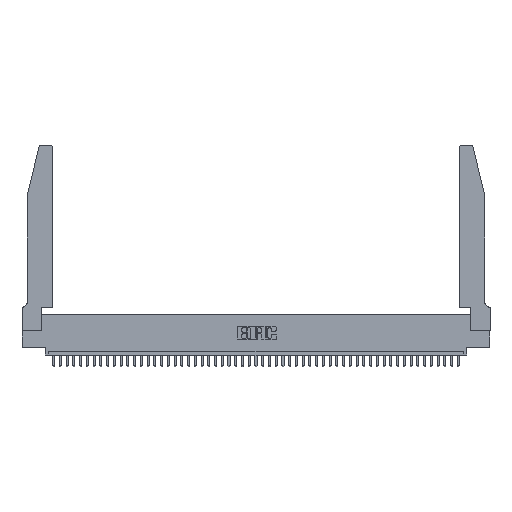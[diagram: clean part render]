
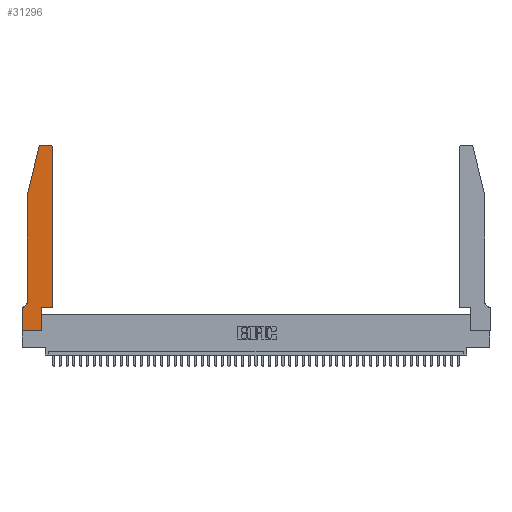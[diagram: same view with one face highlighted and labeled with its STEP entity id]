
A CAD part, top view. The second image highlights one B-rep face of the part: STEP entity #31296.
In plain terms, the highlighted planar face has unit normal (0, 0, 1).
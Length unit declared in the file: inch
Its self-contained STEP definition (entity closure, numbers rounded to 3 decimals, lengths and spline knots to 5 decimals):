
#1289 = DIRECTION ( 'NONE',  ( 1., 0., 0. ) ) ;
#2244 = VECTOR ( 'NONE', #34285, 39.37008 ) ;
#2456 = CARTESIAN_POINT ( 'NONE',  ( 0.2865, 0.35, 0.37 ) ) ;
#2849 = VERTEX_POINT ( 'NONE', #4525 ) ;
#4393 = VECTOR ( 'NONE', #13581, 39.37008 ) ;
#4525 = CARTESIAN_POINT ( 'NONE',  ( 0.0755, 0.42, 0.37 ) ) ;
#4713 = ORIENTED_EDGE ( 'NONE', *, *, #5878, .T. ) ;
#4777 = DIRECTION ( 'NONE',  ( -1., 0., 0. ) ) ;
#5356 = EDGE_CURVE ( 'NONE', #40890, #43727, #7266, .T. ) ;
#5733 = CARTESIAN_POINT ( 'NONE',  ( 0.4505, 0.35, 0.37 ) ) ;
#5854 = CARTESIAN_POINT ( 'NONE',  ( 0.2865, 0.35, 0.37 ) ) ;
#5878 = EDGE_CURVE ( 'NONE', #46808, #28588, #6631, .T. ) ;
#6199 = CARTESIAN_POINT ( 'NONE',  ( 0.4205, 2.72, 0.37 ) ) ;
#6631 = CIRCLE ( 'NONE', #45291, 0.03 ) ;
#7266 = CIRCLE ( 'NONE', #42151, 0.03 ) ;
#7638 = CARTESIAN_POINT ( 'NONE',  ( 0.0055, 0.35, 0.37 ) ) ;
#8181 = VERTEX_POINT ( 'NONE', #22302 ) ;
#9485 = EDGE_CURVE ( 'NONE', #19418, #20852, #24238, .T. ) ;
#9542 = EDGE_CURVE ( 'NONE', #43727, #31948, #17871, .T. ) ;
#10158 = CARTESIAN_POINT ( 'NONE',  ( 0.0755, 0.35, 0.37 ) ) ;
#10326 = DIRECTION ( 'NONE',  ( -1., 0., 0. ) ) ;
#10355 = VECTOR ( 'NONE', #28546, 39.37008 ) ;
#12191 = DIRECTION ( 'NONE',  ( 0., 0., -1. ) ) ;
#12294 = CARTESIAN_POINT ( 'NONE',  ( 0., 0., 0.37 ) ) ;
#12465 = AXIS2_PLACEMENT_3D ( 'NONE', #12862, #12191, #4777 ) ;
#12616 = LINE ( 'NONE', #31312, #34798 ) ;
#12862 = CARTESIAN_POINT ( 'NONE',  ( 0.0055, 0.42, 0.37 ) ) ;
#13145 = VERTEX_POINT ( 'NONE', #36348 ) ;
#13581 = DIRECTION ( 'NONE',  ( -0.239, -0.971, 0. ) ) ;
#13798 = CARTESIAN_POINT ( 'NONE',  ( 0.4205, 2.75, 0.37 ) ) ;
#13918 = CARTESIAN_POINT ( 'NONE',  ( 0.4505, 2.72, 0.37 ) ) ;
#14102 = ORIENTED_EDGE ( 'NONE', *, *, #44651, .T. ) ;
#14173 = ORIENTED_EDGE ( 'NONE', *, *, #23228, .T. ) ;
#15667 = PLANE ( 'NONE',  #28761 ) ;
#15898 = CARTESIAN_POINT ( 'NONE',  ( 0.0755, 2., 0.37 ) ) ;
#16308 = VERTEX_POINT ( 'NONE', #47112 ) ;
#16496 = DIRECTION ( 'NONE',  ( 0., 1., 0. ) ) ;
#16589 = EDGE_CURVE ( 'NONE', #8181, #46808, #12616, .T. ) ;
#16779 = DIRECTION ( 'NONE',  ( 1., 0., 0. ) ) ;
#16995 = FACE_OUTER_BOUND ( 'NONE', #36364, .T. ) ;
#17043 = ORIENTED_EDGE ( 'NONE', *, *, #30662, .T. ) ;
#17255 = DIRECTION ( 'NONE',  ( 0., 0., 1. ) ) ;
#17536 = DIRECTION ( 'NONE',  ( 1., 0., 0. ) ) ;
#17871 = LINE ( 'NONE', #28376, #4393 ) ;
#18011 = DIRECTION ( 'NONE',  ( 0., 0., 1. ) ) ;
#18640 = CARTESIAN_POINT ( 'NONE',  ( 0., 0.35, 0.37 ) ) ;
#18969 = CARTESIAN_POINT ( 'NONE',  ( 0.2605, 2.75, 0.37 ) ) ;
#19367 = CIRCLE ( 'NONE', #12465, 0.07 ) ;
#19418 = VERTEX_POINT ( 'NONE', #19504 ) ;
#19504 = CARTESIAN_POINT ( 'NONE',  ( 0.2865, 0., 0.37 ) ) ;
#19822 = EDGE_CURVE ( 'NONE', #13145, #19418, #47623, .T. ) ;
#20852 = VERTEX_POINT ( 'NONE', #5854 ) ;
#20924 = LINE ( 'NONE', #12294, #2244 ) ;
#21621 = EDGE_CURVE ( 'NONE', #20852, #8181, #23454, .T. ) ;
#22048 = CARTESIAN_POINT ( 'NONE',  ( 0.0755, 2., 0.37 ) ) ;
#22162 = ORIENTED_EDGE ( 'NONE', *, *, #21621, .T. ) ;
#22302 = CARTESIAN_POINT ( 'NONE',  ( 0.4505, 0.35, 0.37 ) ) ;
#22874 = DIRECTION ( 'NONE',  ( -1., 0., 0. ) ) ;
#23228 = EDGE_CURVE ( 'NONE', #28588, #40890, #34170, .T. ) ;
#23454 = LINE ( 'NONE', #5733, #32260 ) ;
#24238 = LINE ( 'NONE', #2456, #10355 ) ;
#25242 = EDGE_CURVE ( 'NONE', #31948, #2849, #29358, .T. ) ;
#28224 = EDGE_CURVE ( 'NONE', #16308, #13145, #20924, .T. ) ;
#28376 = CARTESIAN_POINT ( 'NONE',  ( 0.0755, 2., 0.37 ) ) ;
#28546 = DIRECTION ( 'NONE',  ( 0., 1., 0. ) ) ;
#28588 = VERTEX_POINT ( 'NONE', #13798 ) ;
#28761 = AXIS2_PLACEMENT_3D ( 'NONE', #18640, #44484, #36973 ) ;
#29358 = LINE ( 'NONE', #15898, #41555 ) ;
#30662 = EDGE_CURVE ( 'NONE', #2849, #39352, #19367, .T. ) ;
#30840 = CARTESIAN_POINT ( 'NONE',  ( 0.284, 2.75, 0.37 ) ) ;
#30860 = ORIENTED_EDGE ( 'NONE', *, *, #19822, .T. ) ;
#31014 = CARTESIAN_POINT ( 'NONE',  ( 0.25487, 2.72718, 0.37 ) ) ;
#31296 = ADVANCED_FACE ( 'NONE', ( #16995 ), #15667, .T. ) ;
#31312 = CARTESIAN_POINT ( 'NONE',  ( 0.4505, 0.35, 0.37 ) ) ;
#31948 = VERTEX_POINT ( 'NONE', #22048 ) ;
#32185 = ORIENTED_EDGE ( 'NONE', *, *, #28224, .T. ) ;
#32260 = VECTOR ( 'NONE', #1289, 39.37008 ) ;
#33387 = CARTESIAN_POINT ( 'NONE',  ( 0.284, 2.72, 0.37 ) ) ;
#34170 = LINE ( 'NONE', #18969, #36563 ) ;
#34285 = DIRECTION ( 'NONE',  ( 0., -1., 0. ) ) ;
#34398 = VECTOR ( 'NONE', #10326, 39.37008 ) ;
#34798 = VECTOR ( 'NONE', #16496, 39.37008 ) ;
#36348 = CARTESIAN_POINT ( 'NONE',  ( 0., 0., 0.37 ) ) ;
#36364 = EDGE_LOOP ( 'NONE', ( #14173, #40744, #37328, #46844, #17043, #14102, #32185, #30860, #37167, #22162, #38409, #4713 ) ) ;
#36525 = VECTOR ( 'NONE', #38486, 39.37008 ) ;
#36563 = VECTOR ( 'NONE', #22874, 39.37008 ) ;
#36973 = DIRECTION ( 'NONE',  ( 1., 0., 0. ) ) ;
#37167 = ORIENTED_EDGE ( 'NONE', *, *, #9485, .T. ) ;
#37328 = ORIENTED_EDGE ( 'NONE', *, *, #9542, .T. ) ;
#38145 = CARTESIAN_POINT ( 'NONE',  ( 0., 0., 0.37 ) ) ;
#38409 = ORIENTED_EDGE ( 'NONE', *, *, #16589, .T. ) ;
#38486 = DIRECTION ( 'NONE',  ( 1., 0., 0. ) ) ;
#39352 = VERTEX_POINT ( 'NONE', #7638 ) ;
#40744 = ORIENTED_EDGE ( 'NONE', *, *, #5356, .T. ) ;
#40890 = VERTEX_POINT ( 'NONE', #30840 ) ;
#41555 = VECTOR ( 'NONE', #42284, 39.37008 ) ;
#42151 = AXIS2_PLACEMENT_3D ( 'NONE', #33387, #18011, #17536 ) ;
#42284 = DIRECTION ( 'NONE',  ( 0., -1., 0. ) ) ;
#43727 = VERTEX_POINT ( 'NONE', #31014 ) ;
#44484 = DIRECTION ( 'NONE',  ( 0., 0., 1. ) ) ;
#44651 = EDGE_CURVE ( 'NONE', #39352, #16308, #46704, .T. ) ;
#45291 = AXIS2_PLACEMENT_3D ( 'NONE', #6199, #17255, #16779 ) ;
#46704 = LINE ( 'NONE', #10158, #34398 ) ;
#46808 = VERTEX_POINT ( 'NONE', #13918 ) ;
#46844 = ORIENTED_EDGE ( 'NONE', *, *, #25242, .T. ) ;
#47112 = CARTESIAN_POINT ( 'NONE',  ( 0., 0.35, 0.37 ) ) ;
#47623 = LINE ( 'NONE', #38145, #36525 ) ;
